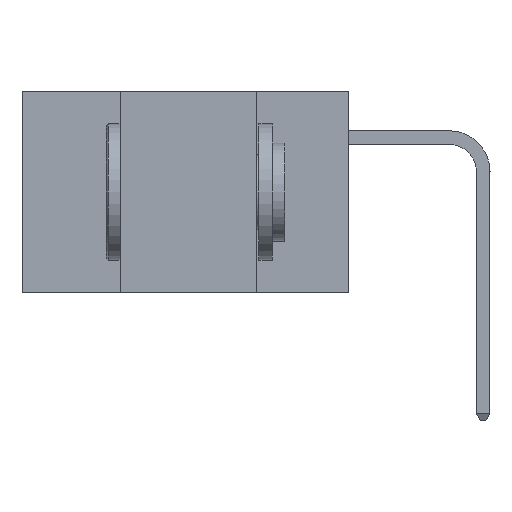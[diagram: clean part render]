
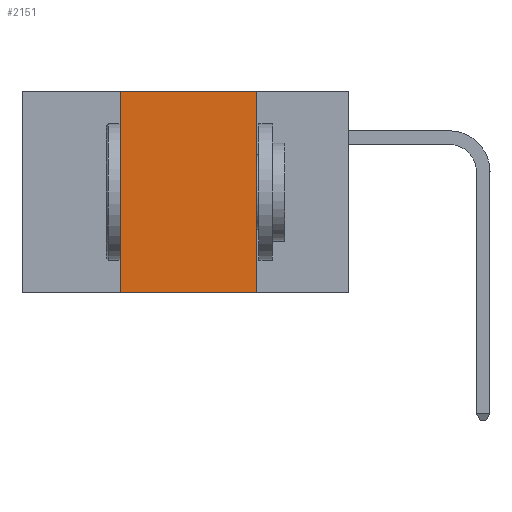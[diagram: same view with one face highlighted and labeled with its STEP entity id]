
A CAD part, left-side view. The second image highlights one B-rep face of the part: STEP entity #2151.
In plain terms, the highlighted planar face has unit normal (-1, 0, 0).
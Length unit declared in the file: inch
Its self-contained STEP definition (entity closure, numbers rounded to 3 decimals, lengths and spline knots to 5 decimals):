
#65 = VECTOR ( 'NONE', #13387, 39.37008 ) ;
#212 = VECTOR ( 'NONE', #4210, 39.37008 ) ;
#287 = CARTESIAN_POINT ( 'NONE',  ( 0., 0.17, 0. ) ) ;
#2151 = ADVANCED_FACE ( 'NONE', ( #13971 ), #4043, .F. ) ;
#2628 = VERTEX_POINT ( 'NONE', #15111 ) ;
#2714 = DIRECTION ( 'NONE',  ( 0., -1., 0. ) ) ;
#3292 = LINE ( 'NONE', #11907, #16282 ) ;
#3434 = EDGE_LOOP ( 'NONE', ( #8412, #12212, #15431, #13373 ) ) ;
#3931 = DIRECTION ( 'NONE',  ( 0., 0., -1. ) ) ;
#3985 = DIRECTION ( 'NONE',  ( 1., 0., 0. ) ) ;
#4043 = PLANE ( 'NONE',  #5529 ) ;
#4210 = DIRECTION ( 'NONE',  ( 0., 0., -1. ) ) ;
#4226 = CARTESIAN_POINT ( 'NONE',  ( 0., 0.6, 0. ) ) ;
#5286 = CARTESIAN_POINT ( 'NONE',  ( 0., 0.17, -0.37 ) ) ;
#5529 = AXIS2_PLACEMENT_3D ( 'NONE', #4226, #3985, #3931 ) ;
#6016 = CARTESIAN_POINT ( 'NONE',  ( 0., 0.17, 0. ) ) ;
#6754 = LINE ( 'NONE', #287, #212 ) ;
#7763 = CARTESIAN_POINT ( 'NONE',  ( 0., 0.42, 0. ) ) ;
#8093 = DIRECTION ( 'NONE',  ( 0., 0., 1. ) ) ;
#8348 = LINE ( 'NONE', #9181, #14616 ) ;
#8412 = ORIENTED_EDGE ( 'NONE', *, *, #14521, .F. ) ;
#8900 = VERTEX_POINT ( 'NONE', #7763 ) ;
#8946 = VERTEX_POINT ( 'NONE', #5286 ) ;
#9181 = CARTESIAN_POINT ( 'NONE',  ( 0., 0.6, -0.37 ) ) ;
#9672 = CARTESIAN_POINT ( 'NONE',  ( 0., 0.6, 0. ) ) ;
#11907 = CARTESIAN_POINT ( 'NONE',  ( 0., 0.42, 0. ) ) ;
#12212 = ORIENTED_EDGE ( 'NONE', *, *, #12507, .F. ) ;
#12507 = EDGE_CURVE ( 'NONE', #8900, #15594, #13735, .T. ) ;
#13373 = ORIENTED_EDGE ( 'NONE', *, *, #14427, .T. ) ;
#13387 = DIRECTION ( 'NONE',  ( 0., -1., 0. ) ) ;
#13735 = LINE ( 'NONE', #9672, #65 ) ;
#13971 = FACE_OUTER_BOUND ( 'NONE', #3434, .T. ) ;
#14427 = EDGE_CURVE ( 'NONE', #2628, #8946, #8348, .T. ) ;
#14519 = EDGE_CURVE ( 'NONE', #2628, #8900, #3292, .T. ) ;
#14521 = EDGE_CURVE ( 'NONE', #15594, #8946, #6754, .T. ) ;
#14616 = VECTOR ( 'NONE', #2714, 39.37008 ) ;
#15111 = CARTESIAN_POINT ( 'NONE',  ( 0., 0.42, -0.37 ) ) ;
#15431 = ORIENTED_EDGE ( 'NONE', *, *, #14519, .F. ) ;
#15594 = VERTEX_POINT ( 'NONE', #6016 ) ;
#16282 = VECTOR ( 'NONE', #8093, 39.37008 ) ;
